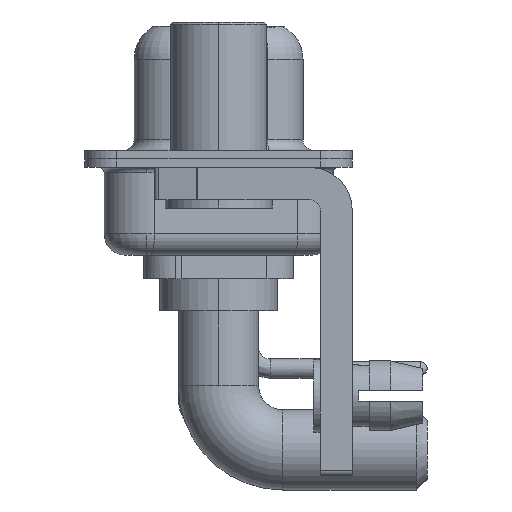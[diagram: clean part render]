
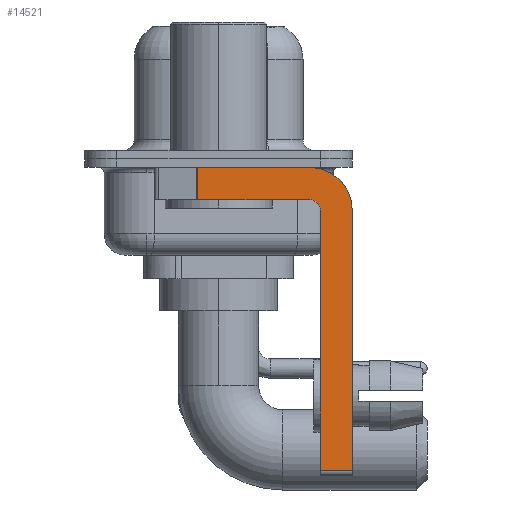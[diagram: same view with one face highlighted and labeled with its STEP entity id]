
A CAD part, left-side view. The second image highlights one B-rep face of the part: STEP entity #14521.
In plain terms, the highlighted planar face has unit normal (-1, 0, 0).
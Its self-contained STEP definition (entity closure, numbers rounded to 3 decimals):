
#40 = CARTESIAN_POINT ( 'NONE',  ( -2.9, -4.25, -1.9 ) ) ;
#229 = VERTEX_POINT ( 'NONE', #2839 ) ;
#276 = LINE ( 'NONE', #40, #502 ) ;
#502 = VECTOR ( 'NONE', #3269, 1000. ) ;
#703 = VERTEX_POINT ( 'NONE', #17097 ) ;
#1095 = CARTESIAN_POINT ( 'NONE',  ( -2.9, -4.75, -14.8 ) ) ;
#1280 = LINE ( 'NONE', #8287, #1951 ) ;
#1452 = CIRCLE ( 'NONE', #5845, 0.5 ) ;
#1951 = VECTOR ( 'NONE', #15257, 1000. ) ;
#2176 = EDGE_CURVE ( 'NONE', #18644, #3019, #1280, .T. ) ;
#2839 = CARTESIAN_POINT ( 'NONE',  ( -2.9, -4.75, -2.4 ) ) ;
#3019 = VERTEX_POINT ( 'NONE', #18069 ) ;
#3269 = DIRECTION ( 'NONE',  ( 0., 1., 0. ) ) ;
#4454 = EDGE_CURVE ( 'NONE', #10828, #5528, #19898, .T. ) ;
#4569 = CARTESIAN_POINT ( 'NONE',  ( -2.9, -6.25, -2.4 ) ) ;
#4882 = ORIENTED_EDGE ( 'NONE', *, *, #4454, .F. ) ;
#4890 = DIRECTION ( 'NONE',  ( 0., 0., -1. ) ) ;
#4954 = VECTOR ( 'NONE', #5787, 1000. ) ;
#5181 = DIRECTION ( 'NONE',  ( 0., 0., 1. ) ) ;
#5370 = CIRCLE ( 'NONE', #14879, 2. ) ;
#5517 = EDGE_CURVE ( 'NONE', #11370, #229, #14732, .T. ) ;
#5528 = VERTEX_POINT ( 'NONE', #18048 ) ;
#5787 = DIRECTION ( 'NONE',  ( 0., 0., 1. ) ) ;
#5845 = AXIS2_PLACEMENT_3D ( 'NONE', #15596, #13884, #5181 ) ;
#6331 = CARTESIAN_POINT ( 'NONE',  ( -2.9, 0.978, -1.9 ) ) ;
#6818 = PLANE ( 'NONE',  #12785 ) ;
#8287 = CARTESIAN_POINT ( 'NONE',  ( -2.9, 3., -0.4 ) ) ;
#8393 = EDGE_CURVE ( 'NONE', #11370, #5528, #22072, .T. ) ;
#8449 = CARTESIAN_POINT ( 'NONE',  ( -2.9, -4.25, -2.4 ) ) ;
#9477 = EDGE_CURVE ( 'NONE', #18644, #703, #13211, .T. ) ;
#9574 = DIRECTION ( 'NONE',  ( 0., 0., -1. ) ) ;
#10828 = VERTEX_POINT ( 'NONE', #17786 ) ;
#10947 = CARTESIAN_POINT ( 'NONE',  ( -2.9, -4.25, -1.9 ) ) ;
#11273 = ORIENTED_EDGE ( 'NONE', *, *, #15110, .F. ) ;
#11370 = VERTEX_POINT ( 'NONE', #22140 ) ;
#11641 = VECTOR ( 'NONE', #11694, 1000. ) ;
#11694 = DIRECTION ( 'NONE',  ( 0., -1., 0. ) ) ;
#11726 = VERTEX_POINT ( 'NONE', #10947 ) ;
#11865 = EDGE_CURVE ( 'NONE', #3019, #10828, #5370, .T. ) ;
#12785 = AXIS2_PLACEMENT_3D ( 'NONE', #8449, #15310, #4890 ) ;
#13211 = LINE ( 'NONE', #6331, #15704 ) ;
#13884 = DIRECTION ( 'NONE',  ( -1., 0., 0. ) ) ;
#14521 = ADVANCED_FACE ( 'NONE', ( #22586 ), #6818, .F. ) ;
#14535 = DIRECTION ( 'NONE',  ( 0., 0., -1. ) ) ;
#14732 = LINE ( 'NONE', #1095, #4954 ) ;
#14768 = ORIENTED_EDGE ( 'NONE', *, *, #8393, .T. ) ;
#14879 = AXIS2_PLACEMENT_3D ( 'NONE', #22225, #20523, #9574 ) ;
#14976 = ORIENTED_EDGE ( 'NONE', *, *, #21771, .F. ) ;
#15110 = EDGE_CURVE ( 'NONE', #229, #11726, #1452, .T. ) ;
#15257 = DIRECTION ( 'NONE',  ( 0., -1., 0. ) ) ;
#15310 = DIRECTION ( 'NONE',  ( 1., 0., 0. ) ) ;
#15596 = CARTESIAN_POINT ( 'NONE',  ( -2.9, -4.25, -2.4 ) ) ;
#15704 = VECTOR ( 'NONE', #16652, 1000. ) ;
#15753 = CARTESIAN_POINT ( 'NONE',  ( -2.9, 0.978, -0.4 ) ) ;
#16294 = ORIENTED_EDGE ( 'NONE', *, *, #11865, .F. ) ;
#16652 = DIRECTION ( 'NONE',  ( 0., 0., -1. ) ) ;
#16875 = ORIENTED_EDGE ( 'NONE', *, *, #9477, .T. ) ;
#17097 = CARTESIAN_POINT ( 'NONE',  ( -2.9, 0.978, -1.9 ) ) ;
#17786 = CARTESIAN_POINT ( 'NONE',  ( -2.9, -6.25, -2.4 ) ) ;
#18048 = CARTESIAN_POINT ( 'NONE',  ( -2.9, -6.25, -14.55 ) ) ;
#18069 = CARTESIAN_POINT ( 'NONE',  ( -2.9, -4.25, -0.4 ) ) ;
#18211 = ORIENTED_EDGE ( 'NONE', *, *, #5517, .F. ) ;
#18644 = VERTEX_POINT ( 'NONE', #15753 ) ;
#18784 = VECTOR ( 'NONE', #14535, 1000. ) ;
#19339 = ORIENTED_EDGE ( 'NONE', *, *, #2176, .F. ) ;
#19898 = LINE ( 'NONE', #4569, #18784 ) ;
#20256 = CARTESIAN_POINT ( 'NONE',  ( -2.9, -4.25, -14.55 ) ) ;
#20523 = DIRECTION ( 'NONE',  ( 1., 0., 0. ) ) ;
#20731 = EDGE_LOOP ( 'NONE', ( #19339, #16875, #14976, #11273, #18211, #14768, #4882, #16294 ) ) ;
#21771 = EDGE_CURVE ( 'NONE', #11726, #703, #276, .T. ) ;
#22072 = LINE ( 'NONE', #20256, #11641 ) ;
#22140 = CARTESIAN_POINT ( 'NONE',  ( -2.9, -4.75, -14.55 ) ) ;
#22225 = CARTESIAN_POINT ( 'NONE',  ( -2.9, -4.25, -2.4 ) ) ;
#22586 = FACE_OUTER_BOUND ( 'NONE', #20731, .T. ) ;
